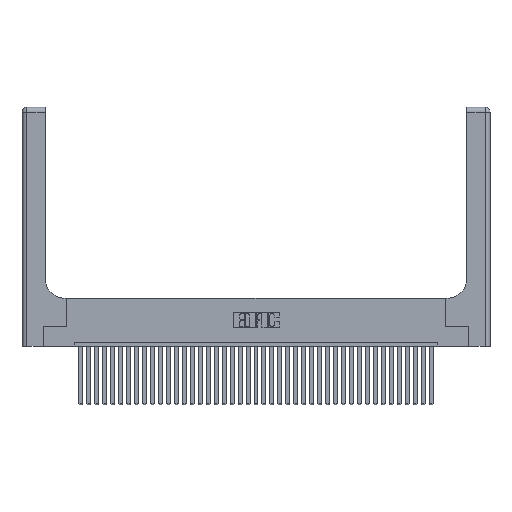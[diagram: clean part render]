
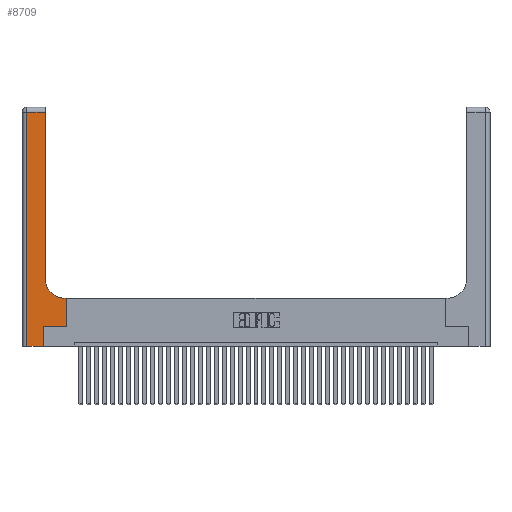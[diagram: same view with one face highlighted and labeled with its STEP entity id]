
A CAD part, top view. The second image highlights one B-rep face of the part: STEP entity #8709.
In plain terms, the highlighted planar face has unit normal (0, 0, 1).
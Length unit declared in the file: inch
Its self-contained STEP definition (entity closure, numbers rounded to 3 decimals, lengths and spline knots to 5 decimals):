
#465 = VECTOR ( 'NONE', #35023, 39.37008 ) ;
#1948 = ORIENTED_EDGE ( 'NONE', *, *, #26413, .T. ) ;
#2221 = DIRECTION ( 'NONE',  ( -1., 0., 0. ) ) ;
#2303 = DIRECTION ( 'NONE',  ( -1., 0., 0. ) ) ;
#3588 = VECTOR ( 'NONE', #29073, 39.37008 ) ;
#3789 = VECTOR ( 'NONE', #31078, 39.37008 ) ;
#3950 = DIRECTION ( 'NONE',  ( 0., 0., -1. ) ) ;
#4388 = EDGE_CURVE ( 'NONE', #29144, #22257, #11922, .T. ) ;
#4513 = DIRECTION ( 'NONE',  ( -1., 0., 0. ) ) ;
#4908 = VECTOR ( 'NONE', #8867, 39.37008 ) ;
#5163 = VERTEX_POINT ( 'NONE', #21499 ) ;
#5362 = EDGE_CURVE ( 'NONE', #22257, #11388, #7231, .T. ) ;
#5379 = VERTEX_POINT ( 'NONE', #19954 ) ;
#5719 = CARTESIAN_POINT ( 'NONE',  ( 0.5585, 0.25, 0.37 ) ) ;
#5988 = CARTESIAN_POINT ( 'NONE',  ( 0.269, 0.25, 0.37 ) ) ;
#5989 = AXIS2_PLACEMENT_3D ( 'NONE', #36929, #7360, #4513 ) ;
#6624 = EDGE_LOOP ( 'NONE', ( #31980, #14654, #8110, #31257, #24636, #19437, #8673, #1948, #18833 ) ) ;
#6680 = LINE ( 'NONE', #21490, #18677 ) ;
#7105 = CARTESIAN_POINT ( 'NONE',  ( 0., 0., 0.37 ) ) ;
#7231 = LINE ( 'NONE', #14028, #27638 ) ;
#7360 = DIRECTION ( 'NONE',  ( 0., 0., -1. ) ) ;
#8049 = EDGE_CURVE ( 'NONE', #22275, #20476, #11690, .T. ) ;
#8110 = ORIENTED_EDGE ( 'NONE', *, *, #29839, .T. ) ;
#8212 = CARTESIAN_POINT ( 'NONE',  ( 0.2915, 2.94, 0.37 ) ) ;
#8673 = ORIENTED_EDGE ( 'NONE', *, *, #9854, .T. ) ;
#8709 = ADVANCED_FACE ( 'NONE', ( #27516 ), #13281, .F. ) ;
#8867 = DIRECTION ( 'NONE',  ( 0., -1., 0. ) ) ;
#9479 = EDGE_CURVE ( 'NONE', #24894, #29144, #10776, .T. ) ;
#9854 = EDGE_CURVE ( 'NONE', #20476, #5379, #26072, .T. ) ;
#10258 = VECTOR ( 'NONE', #23385, 39.37008 ) ;
#10776 = CIRCLE ( 'NONE', #11524, 0.25 ) ;
#11205 = CARTESIAN_POINT ( 'NONE',  ( 0.5585, 0.25, 0.37 ) ) ;
#11388 = VERTEX_POINT ( 'NONE', #30551 ) ;
#11524 = AXIS2_PLACEMENT_3D ( 'NONE', #21631, #3950, #24624 ) ;
#11690 = LINE ( 'NONE', #34299, #3789 ) ;
#11922 = LINE ( 'NONE', #16169, #3588 ) ;
#13281 = PLANE ( 'NONE',  #5989 ) ;
#14028 = CARTESIAN_POINT ( 'NONE',  ( 0., 2.94, 0.37 ) ) ;
#14259 = EDGE_CURVE ( 'NONE', #30762, #22275, #6680, .T. ) ;
#14654 = ORIENTED_EDGE ( 'NONE', *, *, #5362, .T. ) ;
#16169 = CARTESIAN_POINT ( 'NONE',  ( 0.2915, 3., 0.37 ) ) ;
#18677 = VECTOR ( 'NONE', #21626, 39.37008 ) ;
#18833 = ORIENTED_EDGE ( 'NONE', *, *, #9479, .T. ) ;
#19357 = EDGE_CURVE ( 'NONE', #5163, #30762, #25561, .T. ) ;
#19392 = LINE ( 'NONE', #20246, #33849 ) ;
#19437 = ORIENTED_EDGE ( 'NONE', *, *, #8049, .T. ) ;
#19954 = CARTESIAN_POINT ( 'NONE',  ( 0.5585, 0.6, 0.37 ) ) ;
#20246 = CARTESIAN_POINT ( 'NONE',  ( 0.2915, 0.6, 0.37 ) ) ;
#20476 = VERTEX_POINT ( 'NONE', #5719 ) ;
#21490 = CARTESIAN_POINT ( 'NONE',  ( 0.269, 0., 0.37 ) ) ;
#21499 = CARTESIAN_POINT ( 'NONE',  ( 0.06, 0., 0.37 ) ) ;
#21626 = DIRECTION ( 'NONE',  ( 0., 1., 0. ) ) ;
#21631 = CARTESIAN_POINT ( 'NONE',  ( 0.5415, 0.85, 0.37 ) ) ;
#22257 = VERTEX_POINT ( 'NONE', #8212 ) ;
#22275 = VERTEX_POINT ( 'NONE', #5988 ) ;
#23385 = DIRECTION ( 'NONE',  ( 1., 0., 0. ) ) ;
#24624 = DIRECTION ( 'NONE',  ( 1., 0., 0. ) ) ;
#24636 = ORIENTED_EDGE ( 'NONE', *, *, #14259, .T. ) ;
#24894 = VERTEX_POINT ( 'NONE', #31189 ) ;
#25561 = LINE ( 'NONE', #7105, #10258 ) ;
#26072 = LINE ( 'NONE', #11205, #465 ) ;
#26413 = EDGE_CURVE ( 'NONE', #5379, #24894, #19392, .T. ) ;
#27516 = FACE_OUTER_BOUND ( 'NONE', #6624, .T. ) ;
#27638 = VECTOR ( 'NONE', #2303, 39.37008 ) ;
#29073 = DIRECTION ( 'NONE',  ( 0., 1., 0. ) ) ;
#29144 = VERTEX_POINT ( 'NONE', #34760 ) ;
#29839 = EDGE_CURVE ( 'NONE', #11388, #5163, #34069, .T. ) ;
#30551 = CARTESIAN_POINT ( 'NONE',  ( 0.06, 2.94, 0.37 ) ) ;
#30762 = VERTEX_POINT ( 'NONE', #31358 ) ;
#31078 = DIRECTION ( 'NONE',  ( 1., 0., 0. ) ) ;
#31189 = CARTESIAN_POINT ( 'NONE',  ( 0.5415, 0.6, 0.37 ) ) ;
#31257 = ORIENTED_EDGE ( 'NONE', *, *, #19357, .T. ) ;
#31358 = CARTESIAN_POINT ( 'NONE',  ( 0.269, 0., 0.37 ) ) ;
#31980 = ORIENTED_EDGE ( 'NONE', *, *, #4388, .T. ) ;
#32370 = CARTESIAN_POINT ( 'NONE',  ( 0.06, 3., 0.37 ) ) ;
#33849 = VECTOR ( 'NONE', #2221, 39.37008 ) ;
#34069 = LINE ( 'NONE', #32370, #4908 ) ;
#34299 = CARTESIAN_POINT ( 'NONE',  ( 0.269, 0.25, 0.37 ) ) ;
#34760 = CARTESIAN_POINT ( 'NONE',  ( 0.2915, 0.85, 0.37 ) ) ;
#35023 = DIRECTION ( 'NONE',  ( 0., 1., 0. ) ) ;
#36929 = CARTESIAN_POINT ( 'NONE',  ( 0., 3., 0.37 ) ) ;
